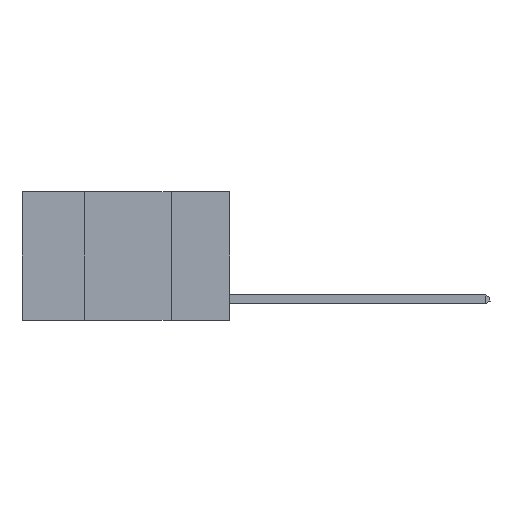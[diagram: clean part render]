
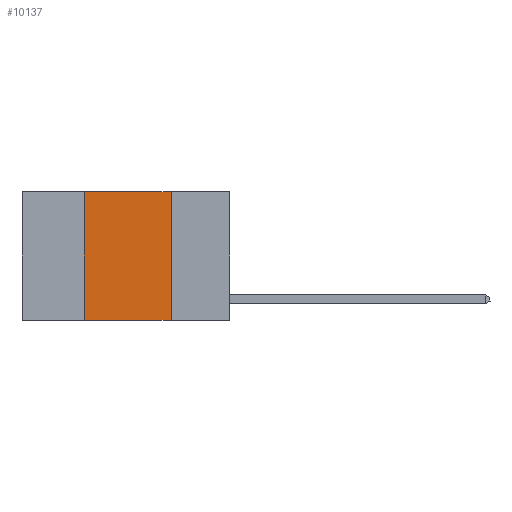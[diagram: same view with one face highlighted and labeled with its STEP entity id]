
A CAD part, left-side view. The second image highlights one B-rep face of the part: STEP entity #10137.
In plain terms, the highlighted planar face has unit normal (-1, 0, 0).
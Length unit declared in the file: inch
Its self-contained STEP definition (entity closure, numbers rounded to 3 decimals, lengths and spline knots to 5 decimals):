
#258 = VECTOR ( 'NONE', #11632, 39.37008 ) ;
#303 = EDGE_CURVE ( 'NONE', #2122, #9457, #9840, .T. ) ;
#420 = DIRECTION ( 'NONE',  ( 0., 0., 1. ) ) ;
#483 = CARTESIAN_POINT ( 'NONE',  ( 0., 0.17, 0. ) ) ;
#1233 = LINE ( 'NONE', #9596, #8601 ) ;
#1332 = CARTESIAN_POINT ( 'NONE',  ( 0., 0.17, -0.37 ) ) ;
#2122 = VERTEX_POINT ( 'NONE', #8146 ) ;
#2242 = AXIS2_PLACEMENT_3D ( 'NONE', #7627, #10519, #9554 ) ;
#2626 = VECTOR ( 'NONE', #11456, 39.37008 ) ;
#3283 = EDGE_LOOP ( 'NONE', ( #3374, #7947, #3545, #9793 ) ) ;
#3374 = ORIENTED_EDGE ( 'NONE', *, *, #10540, .F. ) ;
#3545 = ORIENTED_EDGE ( 'NONE', *, *, #3944, .F. ) ;
#3944 = EDGE_CURVE ( 'NONE', #7784, #2122, #1233, .T. ) ;
#4420 = DIRECTION ( 'NONE',  ( 0., -1., 0. ) ) ;
#4478 = LINE ( 'NONE', #6926, #6980 ) ;
#4884 = LINE ( 'NONE', #4949, #2626 ) ;
#4949 = CARTESIAN_POINT ( 'NONE',  ( 0., 0.17, 0. ) ) ;
#6184 = EDGE_CURVE ( 'NONE', #7784, #9692, #4478, .T. ) ;
#6344 = CARTESIAN_POINT ( 'NONE',  ( 0., 0.6, 0. ) ) ;
#6926 = CARTESIAN_POINT ( 'NONE',  ( 0., 0.6, -0.37 ) ) ;
#6980 = VECTOR ( 'NONE', #4420, 39.37008 ) ;
#7248 = CARTESIAN_POINT ( 'NONE',  ( 0., 0.42, -0.37 ) ) ;
#7627 = CARTESIAN_POINT ( 'NONE',  ( 0., 0.6, 0. ) ) ;
#7784 = VERTEX_POINT ( 'NONE', #7248 ) ;
#7947 = ORIENTED_EDGE ( 'NONE', *, *, #303, .F. ) ;
#8146 = CARTESIAN_POINT ( 'NONE',  ( 0., 0.42, 0. ) ) ;
#8601 = VECTOR ( 'NONE', #420, 39.37008 ) ;
#8728 = PLANE ( 'NONE',  #2242 ) ;
#9457 = VERTEX_POINT ( 'NONE', #483 ) ;
#9497 = FACE_OUTER_BOUND ( 'NONE', #3283, .T. ) ;
#9554 = DIRECTION ( 'NONE',  ( 0., 0., -1. ) ) ;
#9596 = CARTESIAN_POINT ( 'NONE',  ( 0., 0.42, 0. ) ) ;
#9692 = VERTEX_POINT ( 'NONE', #1332 ) ;
#9793 = ORIENTED_EDGE ( 'NONE', *, *, #6184, .T. ) ;
#9840 = LINE ( 'NONE', #6344, #258 ) ;
#10137 = ADVANCED_FACE ( 'NONE', ( #9497 ), #8728, .F. ) ;
#10519 = DIRECTION ( 'NONE',  ( 1., 0., 0. ) ) ;
#10540 = EDGE_CURVE ( 'NONE', #9457, #9692, #4884, .T. ) ;
#11456 = DIRECTION ( 'NONE',  ( 0., 0., -1. ) ) ;
#11632 = DIRECTION ( 'NONE',  ( 0., -1., 0. ) ) ;
